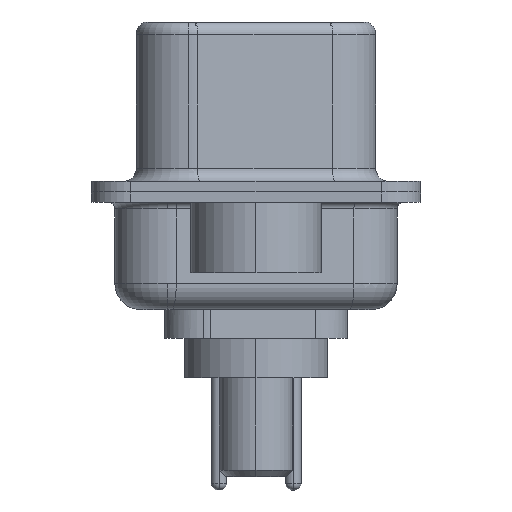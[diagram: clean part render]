
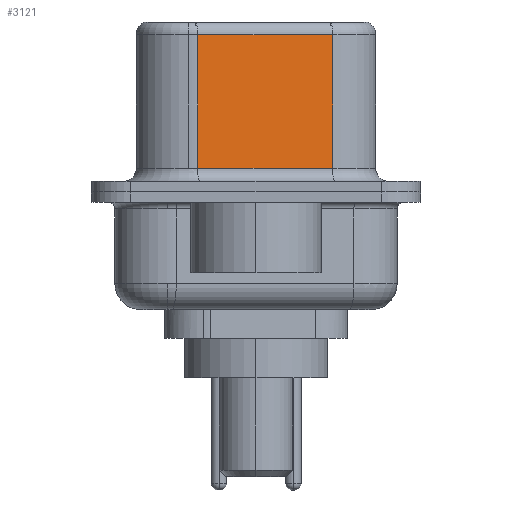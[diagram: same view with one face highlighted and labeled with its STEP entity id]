
A CAD part, left-side view. The second image highlights one B-rep face of the part: STEP entity #3121.
In plain terms, the highlighted planar face has unit normal (-0.985, -0.174, 0).
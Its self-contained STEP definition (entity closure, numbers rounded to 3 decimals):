
#450 = CARTESIAN_POINT ( 'NONE',  ( 4.58, -2.927, 6.52 ) ) ;
#1259 = CARTESIAN_POINT ( 'NONE',  ( 4.58, -2.927, 0.9 ) ) ;
#2077 = VERTEX_POINT ( 'NONE', #3555 ) ;
#3053 = AXIS2_PLACEMENT_3D ( 'NONE', #20923, #5026, #4863 ) ;
#3056 = DIRECTION ( 'NONE',  ( 0.174, -0.985, 0. ) ) ;
#3121 = ADVANCED_FACE ( 'NONE', ( #5239 ), #15556, .F. ) ;
#3555 = CARTESIAN_POINT ( 'NONE',  ( 4.58, -2.927, 6.02 ) ) ;
#3841 = DIRECTION ( 'NONE',  ( 0., 0., -1. ) ) ;
#3999 = CARTESIAN_POINT ( 'NONE',  ( 3.67, 2.233, 6.52 ) ) ;
#4184 = CARTESIAN_POINT ( 'NONE',  ( 3.67, 2.233, 0.9 ) ) ;
#4432 = ORIENTED_EDGE ( 'NONE', *, *, #13916, .F. ) ;
#4760 = LINE ( 'NONE', #450, #17419 ) ;
#4863 = DIRECTION ( 'NONE',  ( -0.174, 0.985, 0. ) ) ;
#5026 = DIRECTION ( 'NONE',  ( 0.985, 0.174, 0. ) ) ;
#5210 = CARTESIAN_POINT ( 'NONE',  ( 4.58, -2.927, 6.02 ) ) ;
#5230 = LINE ( 'NONE', #3999, #16846 ) ;
#5239 = FACE_OUTER_BOUND ( 'NONE', #16165, .T. ) ;
#11835 = VERTEX_POINT ( 'NONE', #1259 ) ;
#11837 = VECTOR ( 'NONE', #16686, 1000. ) ;
#12352 = LINE ( 'NONE', #5210, #11837 ) ;
#12698 = EDGE_CURVE ( 'NONE', #2077, #17516, #12352, .T. ) ;
#13081 = CARTESIAN_POINT ( 'NONE',  ( 4.58, -2.927, 0.9 ) ) ;
#13559 = CARTESIAN_POINT ( 'NONE',  ( 3.67, 2.233, 6.02 ) ) ;
#13916 = EDGE_CURVE ( 'NONE', #2077, #11835, #4760, .T. ) ;
#13992 = DIRECTION ( 'NONE',  ( 0., 0., -1. ) ) ;
#14622 = VECTOR ( 'NONE', #3056, 1000. ) ;
#14813 = VERTEX_POINT ( 'NONE', #4184 ) ;
#14992 = EDGE_CURVE ( 'NONE', #14813, #11835, #17900, .T. ) ;
#15544 = EDGE_CURVE ( 'NONE', #17516, #14813, #5230, .T. ) ;
#15556 = PLANE ( 'NONE',  #3053 ) ;
#16165 = EDGE_LOOP ( 'NONE', ( #4432, #16390, #21183, #16355 ) ) ;
#16355 = ORIENTED_EDGE ( 'NONE', *, *, #14992, .T. ) ;
#16390 = ORIENTED_EDGE ( 'NONE', *, *, #12698, .T. ) ;
#16686 = DIRECTION ( 'NONE',  ( -0.174, 0.985, 0. ) ) ;
#16846 = VECTOR ( 'NONE', #13992, 1000. ) ;
#17419 = VECTOR ( 'NONE', #3841, 1000. ) ;
#17516 = VERTEX_POINT ( 'NONE', #13559 ) ;
#17900 = LINE ( 'NONE', #13081, #14622 ) ;
#20923 = CARTESIAN_POINT ( 'NONE',  ( 4.58, -2.927, 6.52 ) ) ;
#21183 = ORIENTED_EDGE ( 'NONE', *, *, #15544, .T. ) ;
